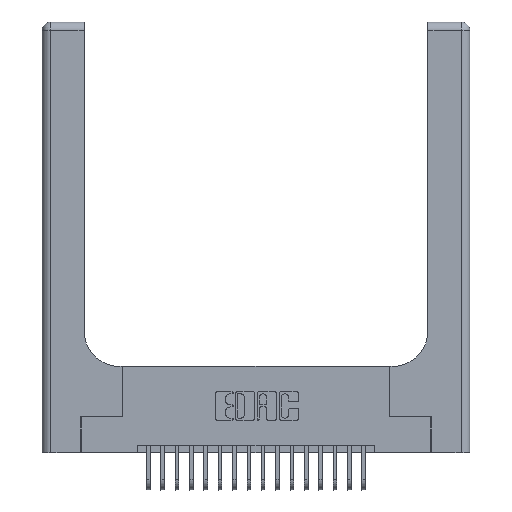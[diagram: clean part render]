
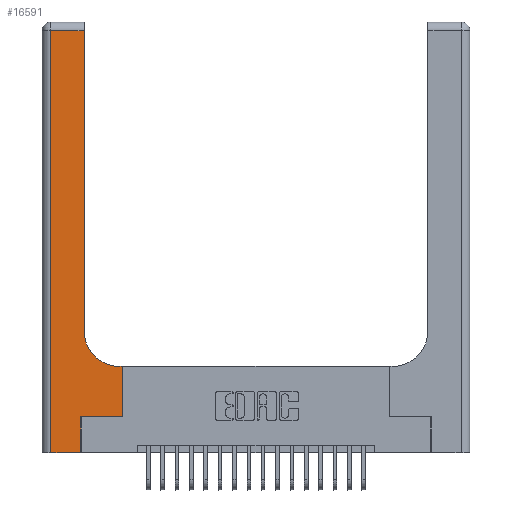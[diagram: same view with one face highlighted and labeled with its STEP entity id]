
A CAD part, top view. The second image highlights one B-rep face of the part: STEP entity #16591.
In plain terms, the highlighted planar face has unit normal (0, 0, 1).
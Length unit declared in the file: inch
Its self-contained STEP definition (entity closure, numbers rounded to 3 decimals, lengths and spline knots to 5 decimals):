
#160 = CARTESIAN_POINT ( 'NONE',  ( 0.2915, 3., 0.37 ) ) ;
#618 = VECTOR ( 'NONE', #6390, 39.37008 ) ;
#1046 = DIRECTION ( 'NONE',  ( 0., 0., -1. ) ) ;
#1080 = EDGE_CURVE ( 'NONE', #19917, #18943, #21805, .T. ) ;
#1249 = CARTESIAN_POINT ( 'NONE',  ( 0.269, 0.25, 0.37 ) ) ;
#1494 = LINE ( 'NONE', #18370, #3413 ) ;
#1738 = EDGE_CURVE ( 'NONE', #18943, #3537, #17315, .T. ) ;
#2199 = LINE ( 'NONE', #14184, #6085 ) ;
#2459 = VECTOR ( 'NONE', #12477, 39.37008 ) ;
#2516 = PLANE ( 'NONE',  #21353 ) ;
#2691 = CARTESIAN_POINT ( 'NONE',  ( 0.269, 0., 0.37 ) ) ;
#2698 = EDGE_LOOP ( 'NONE', ( #4855, #15735, #14577, #17020, #12174, #18326, #7087, #18925, #3257 ) ) ;
#2804 = LINE ( 'NONE', #9913, #13291 ) ;
#2824 = DIRECTION ( 'NONE',  ( -1., 0., 0. ) ) ;
#2878 = VERTEX_POINT ( 'NONE', #15938 ) ;
#3257 = ORIENTED_EDGE ( 'NONE', *, *, #17605, .T. ) ;
#3413 = VECTOR ( 'NONE', #4587, 39.37008 ) ;
#3537 = VERTEX_POINT ( 'NONE', #21745 ) ;
#3792 = VERTEX_POINT ( 'NONE', #11064 ) ;
#4108 = VECTOR ( 'NONE', #5101, 39.37008 ) ;
#4587 = DIRECTION ( 'NONE',  ( 1., 0., 0. ) ) ;
#4855 = ORIENTED_EDGE ( 'NONE', *, *, #12230, .T. ) ;
#5101 = DIRECTION ( 'NONE',  ( 0., 1., 0. ) ) ;
#5433 = FACE_OUTER_BOUND ( 'NONE', #2698, .T. ) ;
#6085 = VECTOR ( 'NONE', #8689, 39.37008 ) ;
#6390 = DIRECTION ( 'NONE',  ( 0., -1., 0. ) ) ;
#6886 = CARTESIAN_POINT ( 'NONE',  ( 0.2915, 2.94, 0.37 ) ) ;
#7074 = CARTESIAN_POINT ( 'NONE',  ( 0.2915, 0.85, 0.37 ) ) ;
#7087 = ORIENTED_EDGE ( 'NONE', *, *, #13509, .T. ) ;
#7376 = CARTESIAN_POINT ( 'NONE',  ( 0.06, 0., 0.37 ) ) ;
#7868 = CARTESIAN_POINT ( 'NONE',  ( 0.269, 0.25, 0.37 ) ) ;
#8146 = CARTESIAN_POINT ( 'NONE',  ( 0., 3., 0.37 ) ) ;
#8332 = VECTOR ( 'NONE', #12827, 39.37008 ) ;
#8689 = DIRECTION ( 'NONE',  ( -1., 0., 0. ) ) ;
#9612 = DIRECTION ( 'NONE',  ( 1., 0., 0. ) ) ;
#9856 = VECTOR ( 'NONE', #9612, 39.37008 ) ;
#9913 = CARTESIAN_POINT ( 'NONE',  ( 0.5585, 0.25, 0.37 ) ) ;
#10855 = EDGE_CURVE ( 'NONE', #15580, #19917, #1494, .T. ) ;
#11064 = CARTESIAN_POINT ( 'NONE',  ( 0.5415, 0.6, 0.37 ) ) ;
#11554 = VERTEX_POINT ( 'NONE', #20979 ) ;
#11721 = CARTESIAN_POINT ( 'NONE',  ( 0.06, 3., 0.37 ) ) ;
#12174 = ORIENTED_EDGE ( 'NONE', *, *, #1080, .T. ) ;
#12230 = EDGE_CURVE ( 'NONE', #20235, #16822, #16625, .T. ) ;
#12477 = DIRECTION ( 'NONE',  ( -1., 0., 0. ) ) ;
#12827 = DIRECTION ( 'NONE',  ( 0., 1., 0. ) ) ;
#13078 = DIRECTION ( 'NONE',  ( 0., 1., 0. ) ) ;
#13291 = VECTOR ( 'NONE', #13078, 39.37008 ) ;
#13509 = EDGE_CURVE ( 'NONE', #3537, #2878, #2804, .T. ) ;
#14184 = CARTESIAN_POINT ( 'NONE',  ( 0.2915, 0.6, 0.37 ) ) ;
#14577 = ORIENTED_EDGE ( 'NONE', *, *, #19431, .T. ) ;
#14936 = DIRECTION ( 'NONE',  ( 1., 0., 0. ) ) ;
#14984 = EDGE_CURVE ( 'NONE', #2878, #3792, #2199, .T. ) ;
#15007 = DIRECTION ( 'NONE',  ( 0., 0., -1. ) ) ;
#15038 = CIRCLE ( 'NONE', #19132, 0.25 ) ;
#15569 = CARTESIAN_POINT ( 'NONE',  ( 0.269, 0., 0.37 ) ) ;
#15579 = EDGE_CURVE ( 'NONE', #16822, #11554, #19285, .T. ) ;
#15580 = VERTEX_POINT ( 'NONE', #7376 ) ;
#15735 = ORIENTED_EDGE ( 'NONE', *, *, #15579, .T. ) ;
#15938 = CARTESIAN_POINT ( 'NONE',  ( 0.5585, 0.6, 0.37 ) ) ;
#16591 = ADVANCED_FACE ( 'NONE', ( #5433 ), #2516, .F. ) ;
#16625 = LINE ( 'NONE', #160, #8332 ) ;
#16822 = VERTEX_POINT ( 'NONE', #6886 ) ;
#17020 = ORIENTED_EDGE ( 'NONE', *, *, #10855, .T. ) ;
#17315 = LINE ( 'NONE', #7868, #9856 ) ;
#17605 = EDGE_CURVE ( 'NONE', #3792, #20235, #15038, .T. ) ;
#18326 = ORIENTED_EDGE ( 'NONE', *, *, #1738, .T. ) ;
#18370 = CARTESIAN_POINT ( 'NONE',  ( 0., 0., 0.37 ) ) ;
#18925 = ORIENTED_EDGE ( 'NONE', *, *, #14984, .T. ) ;
#18943 = VERTEX_POINT ( 'NONE', #1249 ) ;
#19132 = AXIS2_PLACEMENT_3D ( 'NONE', #20119, #15007, #14936 ) ;
#19285 = LINE ( 'NONE', #21448, #2459 ) ;
#19431 = EDGE_CURVE ( 'NONE', #11554, #15580, #21897, .T. ) ;
#19917 = VERTEX_POINT ( 'NONE', #2691 ) ;
#20119 = CARTESIAN_POINT ( 'NONE',  ( 0.5415, 0.85, 0.37 ) ) ;
#20235 = VERTEX_POINT ( 'NONE', #7074 ) ;
#20979 = CARTESIAN_POINT ( 'NONE',  ( 0.06, 2.94, 0.37 ) ) ;
#21353 = AXIS2_PLACEMENT_3D ( 'NONE', #8146, #1046, #2824 ) ;
#21448 = CARTESIAN_POINT ( 'NONE',  ( 0., 2.94, 0.37 ) ) ;
#21745 = CARTESIAN_POINT ( 'NONE',  ( 0.5585, 0.25, 0.37 ) ) ;
#21805 = LINE ( 'NONE', #15569, #4108 ) ;
#21897 = LINE ( 'NONE', #11721, #618 ) ;
